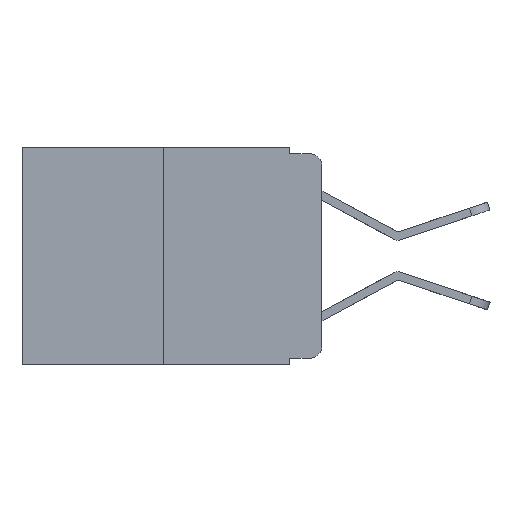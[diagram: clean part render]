
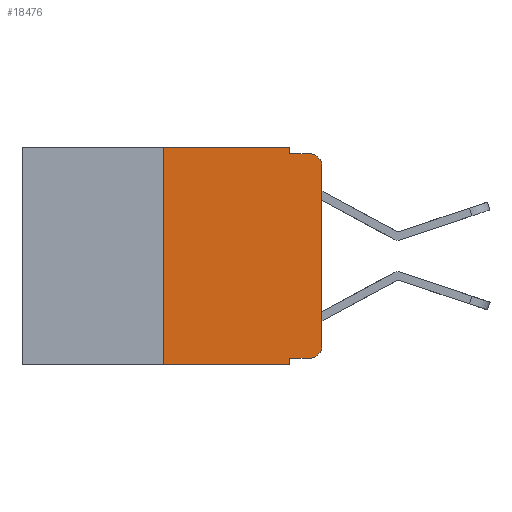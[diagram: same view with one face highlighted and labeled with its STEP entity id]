
A CAD part, left-side view. The second image highlights one B-rep face of the part: STEP entity #18476.
In plain terms, the highlighted planar face has unit normal (-1, 0, 0).
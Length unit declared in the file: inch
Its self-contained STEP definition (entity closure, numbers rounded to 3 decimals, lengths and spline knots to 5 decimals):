
#49 = VERTEX_POINT ( 'NONE', #15155 ) ;
#257 = ORIENTED_EDGE ( 'NONE', *, *, #15423, .F. ) ;
#274 = LINE ( 'NONE', #14469, #15202 ) ;
#704 = DIRECTION ( 'NONE',  ( 0., 0., -1. ) ) ;
#805 = VERTEX_POINT ( 'NONE', #6738 ) ;
#1278 = LINE ( 'NONE', #6406, #14545 ) ;
#1335 = VERTEX_POINT ( 'NONE', #4111 ) ;
#1791 = ORIENTED_EDGE ( 'NONE', *, *, #10638, .F. ) ;
#1907 = AXIS2_PLACEMENT_3D ( 'NONE', #5800, #3834, #20008 ) ;
#2459 = CARTESIAN_POINT ( 'NONE',  ( 0., 0.02, -0.03 ) ) ;
#2460 = ORIENTED_EDGE ( 'NONE', *, *, #8476, .F. ) ;
#2573 = CARTESIAN_POINT ( 'NONE',  ( 0., 0.473, 0. ) ) ;
#2659 = ORIENTED_EDGE ( 'NONE', *, *, #20869, .T. ) ;
#3032 = CIRCLE ( 'NONE', #1907, 0.02 ) ;
#3196 = DIRECTION ( 'NONE',  ( 0., -1., 0. ) ) ;
#3834 = DIRECTION ( 'NONE',  ( -1., 0., 0. ) ) ;
#3865 = DIRECTION ( 'NONE',  ( 0., 0., 1. ) ) ;
#3965 = LINE ( 'NONE', #17704, #19072 ) ;
#4049 = ORIENTED_EDGE ( 'NONE', *, *, #12167, .T. ) ;
#4111 = CARTESIAN_POINT ( 'NONE',  ( 0., 0., -0.313 ) ) ;
#4353 = VERTEX_POINT ( 'NONE', #20207 ) ;
#4416 = DIRECTION ( 'NONE',  ( 0., -1., 0. ) ) ;
#4514 = VECTOR ( 'NONE', #3196, 39.37008 ) ;
#4769 = CARTESIAN_POINT ( 'NONE',  ( 0., 0.473, -0.343 ) ) ;
#5090 = VECTOR ( 'NONE', #20347, 39.37008 ) ;
#5127 = CARTESIAN_POINT ( 'NONE',  ( 0., 0.25, -0.343 ) ) ;
#5562 = LINE ( 'NONE', #9158, #21798 ) ;
#5730 = DIRECTION ( 'NONE',  ( 0., 0., -1. ) ) ;
#5800 = CARTESIAN_POINT ( 'NONE',  ( 0., 0.02, -0.313 ) ) ;
#5897 = CARTESIAN_POINT ( 'NONE',  ( 0., 0., 0. ) ) ;
#6078 = CIRCLE ( 'NONE', #9402, 0.02 ) ;
#6302 = DIRECTION ( 'NONE',  ( 0., -1., 0. ) ) ;
#6406 = CARTESIAN_POINT ( 'NONE',  ( 0., 0.051, 0. ) ) ;
#6470 = VERTEX_POINT ( 'NONE', #12740 ) ;
#6738 = CARTESIAN_POINT ( 'NONE',  ( 0., 0.051, -0.333 ) ) ;
#7259 = PLANE ( 'NONE',  #9371 ) ;
#7271 = EDGE_LOOP ( 'NONE', ( #2659, #12361, #1791, #13767, #2460, #21404, #11548, #257, #4049, #17207 ) ) ;
#8476 = EDGE_CURVE ( 'NONE', #6470, #18996, #16656, .T. ) ;
#9158 = CARTESIAN_POINT ( 'NONE',  ( 0., 0.051, 0. ) ) ;
#9371 = AXIS2_PLACEMENT_3D ( 'NONE', #12717, #10858, #5730 ) ;
#9402 = AXIS2_PLACEMENT_3D ( 'NONE', #2459, #13171, #704 ) ;
#9806 = EDGE_CURVE ( 'NONE', #4353, #16052, #6078, .T. ) ;
#10393 = CARTESIAN_POINT ( 'NONE',  ( 0., 0.051, -0.01 ) ) ;
#10638 = EDGE_CURVE ( 'NONE', #21610, #16052, #20777, .T. ) ;
#10858 = DIRECTION ( 'NONE',  ( 1., 0., 0. ) ) ;
#11548 = ORIENTED_EDGE ( 'NONE', *, *, #16645, .T. ) ;
#12167 = EDGE_CURVE ( 'NONE', #805, #49, #274, .T. ) ;
#12361 = ORIENTED_EDGE ( 'NONE', *, *, #9806, .T. ) ;
#12717 = CARTESIAN_POINT ( 'NONE',  ( 0., 0.473, 0. ) ) ;
#12740 = CARTESIAN_POINT ( 'NONE',  ( 0., 0.25, 0. ) ) ;
#13171 = DIRECTION ( 'NONE',  ( -1., 0., 0. ) ) ;
#13176 = CARTESIAN_POINT ( 'NONE',  ( 0., 0.051, -0.343 ) ) ;
#13767 = ORIENTED_EDGE ( 'NONE', *, *, #20713, .F. ) ;
#13793 = CARTESIAN_POINT ( 'NONE',  ( 0., 0.051, -0.01 ) ) ;
#14230 = FACE_OUTER_BOUND ( 'NONE', #7271, .T. ) ;
#14469 = CARTESIAN_POINT ( 'NONE',  ( 0., 0.051, -0.333 ) ) ;
#14545 = VECTOR ( 'NONE', #16876, 39.37008 ) ;
#14664 = CARTESIAN_POINT ( 'NONE',  ( 0., 0.051, 0. ) ) ;
#14950 = VECTOR ( 'NONE', #4416, 39.37008 ) ;
#15155 = CARTESIAN_POINT ( 'NONE',  ( 0., 0.02, -0.333 ) ) ;
#15202 = VECTOR ( 'NONE', #18410, 39.37008 ) ;
#15423 = EDGE_CURVE ( 'NONE', #805, #21700, #1278, .T. ) ;
#16052 = VERTEX_POINT ( 'NONE', #16371 ) ;
#16371 = CARTESIAN_POINT ( 'NONE',  ( 0., 0.02, -0.01 ) ) ;
#16645 = EDGE_CURVE ( 'NONE', #18734, #21700, #20728, .T. ) ;
#16656 = LINE ( 'NONE', #2573, #21639 ) ;
#16876 = DIRECTION ( 'NONE',  ( 0., 0., -1. ) ) ;
#16891 = EDGE_CURVE ( 'NONE', #49, #1335, #3032, .T. ) ;
#17207 = ORIENTED_EDGE ( 'NONE', *, *, #16891, .T. ) ;
#17704 = CARTESIAN_POINT ( 'NONE',  ( 0., 0.25, 0. ) ) ;
#18224 = EDGE_CURVE ( 'NONE', #18734, #6470, #3965, .T. ) ;
#18241 = LINE ( 'NONE', #5897, #5090 ) ;
#18410 = DIRECTION ( 'NONE',  ( 0., -1., 0. ) ) ;
#18476 = ADVANCED_FACE ( 'NONE', ( #14230 ), #7259, .F. ) ;
#18734 = VERTEX_POINT ( 'NONE', #5127 ) ;
#18996 = VERTEX_POINT ( 'NONE', #14664 ) ;
#19072 = VECTOR ( 'NONE', #3865, 39.37008 ) ;
#20008 = DIRECTION ( 'NONE',  ( 0., 0., -1. ) ) ;
#20207 = CARTESIAN_POINT ( 'NONE',  ( 0., 0., -0.03 ) ) ;
#20347 = DIRECTION ( 'NONE',  ( 0., 0., 1. ) ) ;
#20713 = EDGE_CURVE ( 'NONE', #18996, #21610, #5562, .T. ) ;
#20728 = LINE ( 'NONE', #4769, #14950 ) ;
#20777 = LINE ( 'NONE', #13793, #4514 ) ;
#20869 = EDGE_CURVE ( 'NONE', #1335, #4353, #18241, .T. ) ;
#21404 = ORIENTED_EDGE ( 'NONE', *, *, #18224, .F. ) ;
#21610 = VERTEX_POINT ( 'NONE', #10393 ) ;
#21629 = DIRECTION ( 'NONE',  ( 0., 0., -1. ) ) ;
#21639 = VECTOR ( 'NONE', #6302, 39.37008 ) ;
#21700 = VERTEX_POINT ( 'NONE', #13176 ) ;
#21798 = VECTOR ( 'NONE', #21629, 39.37008 ) ;
